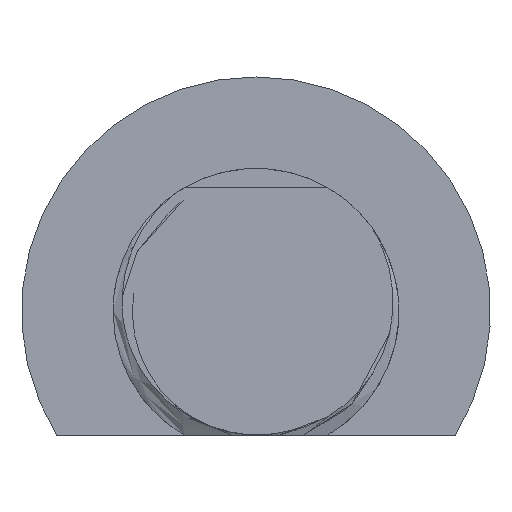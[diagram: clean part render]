
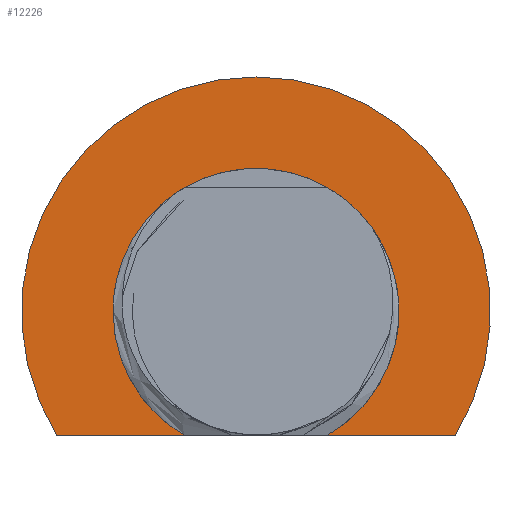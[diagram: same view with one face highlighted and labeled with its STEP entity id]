
A CAD part, front view. The second image highlights one B-rep face of the part: STEP entity #12226.
In plain terms, the highlighted planar face has unit normal (0, -1, 0).
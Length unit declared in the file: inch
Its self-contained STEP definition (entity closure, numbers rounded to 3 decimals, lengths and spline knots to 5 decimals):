
#118 = DIRECTION ( 'NONE',  ( 0., -1., 0. ) ) ;
#626 = VERTEX_POINT ( 'NONE', #10145 ) ;
#724 = CARTESIAN_POINT ( 'NONE',  ( -2.41668, 0.895, 0. ) ) ;
#845 = CARTESIAN_POINT ( 'NONE',  ( -2.2425, 0.895, 0.1081 ) ) ;
#866 = DIRECTION ( 'NONE',  ( 0., 1., 0. ) ) ;
#950 = EDGE_CURVE ( 'NONE', #3673, #2918, #8892, .T. ) ;
#1097 = AXIS2_PLACEMENT_3D ( 'NONE', #6008, #866, #12242 ) ;
#1149 = CARTESIAN_POINT ( 'NONE',  ( -2.06832, 0.895, 0. ) ) ;
#1357 = CARTESIAN_POINT ( 'NONE',  ( -2.17974, 0.895, 0. ) ) ;
#1358 = AXIS2_PLACEMENT_3D ( 'NONE', #12352, #118, #11472 ) ;
#1541 = EDGE_CURVE ( 'NONE', #13133, #2314, #6017, .T. ) ;
#2087 = EDGE_CURVE ( 'NONE', #2918, #2314, #9380, .T. ) ;
#2314 = VERTEX_POINT ( 'NONE', #1149 ) ;
#2385 = EDGE_CURVE ( 'NONE', #6293, #626, #12743, .T. ) ;
#2918 = VERTEX_POINT ( 'NONE', #7222 ) ;
#2985 = LINE ( 'NONE', #3980, #6394 ) ;
#3105 = DIRECTION ( 'NONE',  ( 0., 0., 1. ) ) ;
#3262 = VECTOR ( 'NONE', #12962, 39.37008 ) ;
#3485 = FACE_OUTER_BOUND ( 'NONE', #9640, .T. ) ;
#3673 = VERTEX_POINT ( 'NONE', #724 ) ;
#3979 = CARTESIAN_POINT ( 'NONE',  ( -2.2425, 0.895, 0.1081 ) ) ;
#3980 = CARTESIAN_POINT ( 'NONE',  ( -2.2425, 0.895, 0. ) ) ;
#3995 = DIRECTION ( 'NONE',  ( 0., 0., 1. ) ) ;
#4102 = AXIS2_PLACEMENT_3D ( 'NONE', #3979, #10298, #3105 ) ;
#4301 = DIRECTION ( 'NONE',  ( 0., 0., 1. ) ) ;
#4515 = ORIENTED_EDGE ( 'NONE', *, *, #1541, .T. ) ;
#5015 = AXIS2_PLACEMENT_3D ( 'NONE', #12934, #6018, #10084 ) ;
#5779 = ORIENTED_EDGE ( 'NONE', *, *, #12260, .F. ) ;
#5912 = PLANE ( 'NONE',  #1097 ) ;
#6008 = CARTESIAN_POINT ( 'NONE',  ( -2.2425, 0.895, 0.1081 ) ) ;
#6017 = LINE ( 'NONE', #8867, #3262 ) ;
#6018 = DIRECTION ( 'NONE',  ( 0., 1., 0. ) ) ;
#6026 = DIRECTION ( 'NONE',  ( 0., 1., 0. ) ) ;
#6293 = VERTEX_POINT ( 'NONE', #6874 ) ;
#6394 = VECTOR ( 'NONE', #8220, 39.37008 ) ;
#6419 = DIRECTION ( 'NONE',  ( 0., -1., 0. ) ) ;
#6874 = CARTESIAN_POINT ( 'NONE',  ( -2.3675, 0.895, 0.1081 ) ) ;
#7009 = AXIS2_PLACEMENT_3D ( 'NONE', #845, #6026, #3995 ) ;
#7222 = CARTESIAN_POINT ( 'NONE',  ( -2.2425, 0.895, 0.3131 ) ) ;
#7330 = ORIENTED_EDGE ( 'NONE', *, *, #12905, .T. ) ;
#8210 = CIRCLE ( 'NONE', #4102, 0.125 ) ;
#8220 = DIRECTION ( 'NONE',  ( 1., 0., 0. ) ) ;
#8531 = CARTESIAN_POINT ( 'NONE',  ( -2.1175, 0.895, 0.1081 ) ) ;
#8803 = CIRCLE ( 'NONE', #1358, 0.125 ) ;
#8867 = CARTESIAN_POINT ( 'NONE',  ( -2.2425, 0.895, 0. ) ) ;
#8892 = CIRCLE ( 'NONE', #5015, 0.205 ) ;
#9380 = CIRCLE ( 'NONE', #7009, 0.205 ) ;
#9483 = VERTEX_POINT ( 'NONE', #8531 ) ;
#9568 = AXIS2_PLACEMENT_3D ( 'NONE', #12558, #6419, #4301 ) ;
#9640 = EDGE_LOOP ( 'NONE', ( #10535, #7330, #9834, #5779, #11350, #4515, #10723 ) ) ;
#9834 = ORIENTED_EDGE ( 'NONE', *, *, #2385, .F. ) ;
#9895 = EDGE_CURVE ( 'NONE', #13133, #9483, #8210, .T. ) ;
#10084 = DIRECTION ( 'NONE',  ( 0., 0., 1. ) ) ;
#10145 = CARTESIAN_POINT ( 'NONE',  ( -2.30526, 0.895, 0. ) ) ;
#10298 = DIRECTION ( 'NONE',  ( 0., -1., 0. ) ) ;
#10535 = ORIENTED_EDGE ( 'NONE', *, *, #950, .F. ) ;
#10723 = ORIENTED_EDGE ( 'NONE', *, *, #2087, .F. ) ;
#11350 = ORIENTED_EDGE ( 'NONE', *, *, #9895, .F. ) ;
#11472 = DIRECTION ( 'NONE',  ( 0., 0., 1. ) ) ;
#12226 = ADVANCED_FACE ( 'NONE', ( #3485 ), #5912, .F. ) ;
#12242 = DIRECTION ( 'NONE',  ( 0., 0., 1. ) ) ;
#12260 = EDGE_CURVE ( 'NONE', #9483, #6293, #8803, .T. ) ;
#12352 = CARTESIAN_POINT ( 'NONE',  ( -2.2425, 0.895, 0.1081 ) ) ;
#12558 = CARTESIAN_POINT ( 'NONE',  ( -2.2425, 0.895, 0.1081 ) ) ;
#12743 = CIRCLE ( 'NONE', #9568, 0.125 ) ;
#12905 = EDGE_CURVE ( 'NONE', #3673, #626, #2985, .T. ) ;
#12934 = CARTESIAN_POINT ( 'NONE',  ( -2.2425, 0.895, 0.1081 ) ) ;
#12962 = DIRECTION ( 'NONE',  ( 1., 0., 0. ) ) ;
#13133 = VERTEX_POINT ( 'NONE', #1357 ) ;
